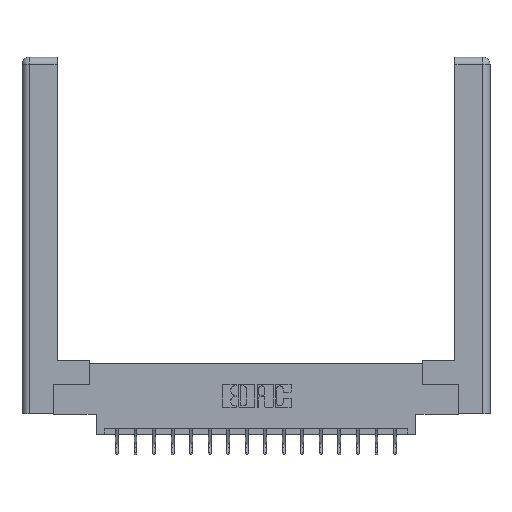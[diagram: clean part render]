
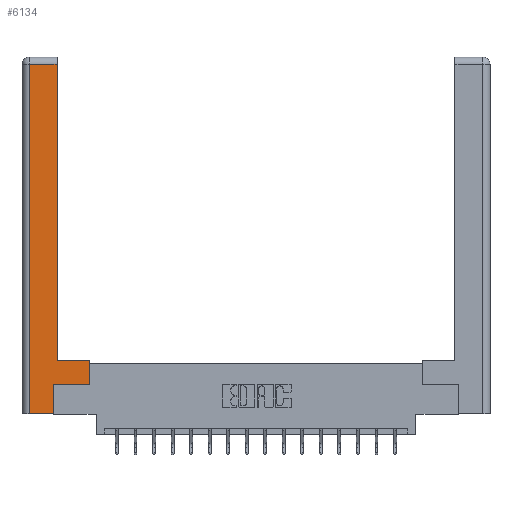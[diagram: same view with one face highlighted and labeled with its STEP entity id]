
A CAD part, top view. The second image highlights one B-rep face of the part: STEP entity #6134.
In plain terms, the highlighted planar face has unit normal (0, 0, 1).
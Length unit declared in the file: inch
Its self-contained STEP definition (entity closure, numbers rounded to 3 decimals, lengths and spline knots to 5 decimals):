
#37 = EDGE_CURVE ( 'NONE', #9254, #11513, #9039, .T. ) ;
#522 = LINE ( 'NONE', #5758, #7518 ) ;
#593 = EDGE_CURVE ( 'NONE', #4674, #9254, #16290, .T. ) ;
#731 = ORIENTED_EDGE ( 'NONE', *, *, #6429, .T. ) ;
#846 = ORIENTED_EDGE ( 'NONE', *, *, #4822, .T. ) ;
#1136 = VECTOR ( 'NONE', #9534, 39.37008 ) ;
#1481 = CARTESIAN_POINT ( 'NONE',  ( 0.265, 0., 0. ) ) ;
#1784 = VERTEX_POINT ( 'NONE', #12136 ) ;
#1976 = FACE_OUTER_BOUND ( 'NONE', #12132, .T. ) ;
#2115 = LINE ( 'NONE', #9164, #7048 ) ;
#2441 = VERTEX_POINT ( 'NONE', #9922 ) ;
#2622 = CARTESIAN_POINT ( 'NONE',  ( 0.565, 0.245, 0. ) ) ;
#3313 = LINE ( 'NONE', #17295, #6693 ) ;
#4283 = DIRECTION ( 'NONE',  ( 0., 1., 0. ) ) ;
#4457 = DIRECTION ( 'NONE',  ( 1., 0., 0. ) ) ;
#4520 = DIRECTION ( 'NONE',  ( 0., 1., 0. ) ) ;
#4674 = VERTEX_POINT ( 'NONE', #12821 ) ;
#4822 = EDGE_CURVE ( 'NONE', #1784, #15712, #7756, .T. ) ;
#5090 = LINE ( 'NONE', #9226, #13715 ) ;
#5147 = ORIENTED_EDGE ( 'NONE', *, *, #13812, .T. ) ;
#5758 = CARTESIAN_POINT ( 'NONE',  ( 0.295, 0.45, 0. ) ) ;
#5821 = DIRECTION ( 'NONE',  ( -1., 0., 0. ) ) ;
#6026 = ORIENTED_EDGE ( 'NONE', *, *, #14576, .T. ) ;
#6134 = ADVANCED_FACE ( 'NONE', ( #1976 ), #13472, .F. ) ;
#6429 = EDGE_CURVE ( 'NONE', #7794, #2441, #3313, .T. ) ;
#6693 = VECTOR ( 'NONE', #4283, 39.37008 ) ;
#7048 = VECTOR ( 'NONE', #12232, 39.37008 ) ;
#7149 = CARTESIAN_POINT ( 'NONE',  ( 0.565, 0.245, 0. ) ) ;
#7321 = ORIENTED_EDGE ( 'NONE', *, *, #593, .T. ) ;
#7480 = ORIENTED_EDGE ( 'NONE', *, *, #18569, .T. ) ;
#7518 = VECTOR ( 'NONE', #5821, 39.37008 ) ;
#7756 = LINE ( 'NONE', #13011, #13446 ) ;
#7794 = VERTEX_POINT ( 'NONE', #10614 ) ;
#7852 = VECTOR ( 'NONE', #15660, 39.37008 ) ;
#7984 = CARTESIAN_POINT ( 'NONE',  ( 0., 0., 0. ) ) ;
#8427 = AXIS2_PLACEMENT_3D ( 'NONE', #7984, #18185, #13864 ) ;
#8749 = CARTESIAN_POINT ( 'NONE',  ( 0.0615, 2.94, 0. ) ) ;
#9039 = LINE ( 'NONE', #18241, #1136 ) ;
#9164 = CARTESIAN_POINT ( 'NONE',  ( 0.0615, 2.94, 0. ) ) ;
#9226 = CARTESIAN_POINT ( 'NONE',  ( 0.0615, 0., 0. ) ) ;
#9254 = VERTEX_POINT ( 'NONE', #7149 ) ;
#9261 = CARTESIAN_POINT ( 'NONE',  ( 0.565, 0.45, 0. ) ) ;
#9534 = DIRECTION ( 'NONE',  ( 0., 1., 0. ) ) ;
#9854 = ORIENTED_EDGE ( 'NONE', *, *, #12960, .T. ) ;
#9922 = CARTESIAN_POINT ( 'NONE',  ( 0.295, 2.94, 0. ) ) ;
#10267 = CARTESIAN_POINT ( 'NONE',  ( 0.265, 0.245, 0. ) ) ;
#10614 = CARTESIAN_POINT ( 'NONE',  ( 0.295, 0.45, 0. ) ) ;
#10907 = VERTEX_POINT ( 'NONE', #8749 ) ;
#11513 = VERTEX_POINT ( 'NONE', #9261 ) ;
#11584 = ORIENTED_EDGE ( 'NONE', *, *, #37, .T. ) ;
#12132 = EDGE_LOOP ( 'NONE', ( #731, #6026, #7480, #846, #9854, #7321, #11584, #5147 ) ) ;
#12136 = CARTESIAN_POINT ( 'NONE',  ( 0.0615, 0., 0. ) ) ;
#12232 = DIRECTION ( 'NONE',  ( -1., 0., 0. ) ) ;
#12821 = CARTESIAN_POINT ( 'NONE',  ( 0.265, 0.245, 0. ) ) ;
#12960 = EDGE_CURVE ( 'NONE', #15712, #4674, #17807, .T. ) ;
#13011 = CARTESIAN_POINT ( 'NONE',  ( 0.265, 0., 0. ) ) ;
#13446 = VECTOR ( 'NONE', #4457, 39.37008 ) ;
#13472 = PLANE ( 'NONE',  #8427 ) ;
#13715 = VECTOR ( 'NONE', #15078, 39.37008 ) ;
#13812 = EDGE_CURVE ( 'NONE', #11513, #7794, #522, .T. ) ;
#13864 = DIRECTION ( 'NONE',  ( -1., 0., 0. ) ) ;
#14576 = EDGE_CURVE ( 'NONE', #2441, #10907, #2115, .T. ) ;
#15078 = DIRECTION ( 'NONE',  ( 0., -1., 0. ) ) ;
#15307 = VECTOR ( 'NONE', #4520, 39.37008 ) ;
#15660 = DIRECTION ( 'NONE',  ( 1., 0., 0. ) ) ;
#15712 = VERTEX_POINT ( 'NONE', #1481 ) ;
#16290 = LINE ( 'NONE', #2622, #7852 ) ;
#17295 = CARTESIAN_POINT ( 'NONE',  ( 0.295, 3., 0. ) ) ;
#17807 = LINE ( 'NONE', #10267, #15307 ) ;
#18185 = DIRECTION ( 'NONE',  ( 0., 0., -1. ) ) ;
#18241 = CARTESIAN_POINT ( 'NONE',  ( 0.565, 0.45, 0. ) ) ;
#18569 = EDGE_CURVE ( 'NONE', #10907, #1784, #5090, .T. ) ;
